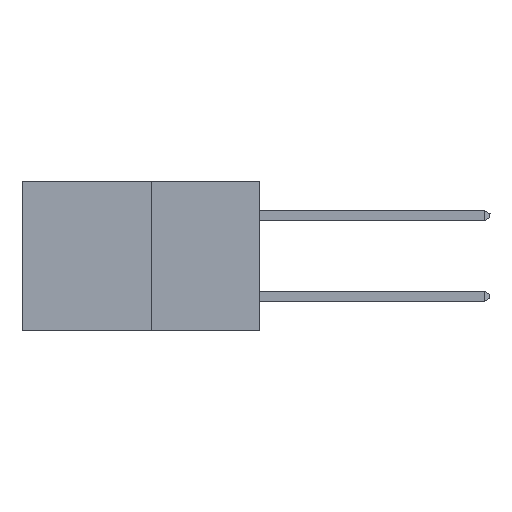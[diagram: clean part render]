
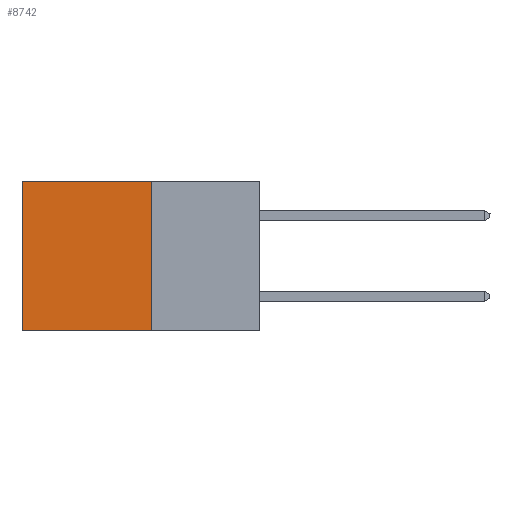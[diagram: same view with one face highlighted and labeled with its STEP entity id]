
A CAD part, left-side view. The second image highlights one B-rep face of the part: STEP entity #8742.
In plain terms, the highlighted planar face has unit normal (-1, 0, 0).
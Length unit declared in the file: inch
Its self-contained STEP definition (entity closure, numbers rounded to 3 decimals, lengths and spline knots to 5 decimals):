
#22 = VECTOR ( 'NONE', #3470, 39.37008 ) ;
#344 = ORIENTED_EDGE ( 'NONE', *, *, #5314, .F. ) ;
#728 = CARTESIAN_POINT ( 'NONE',  ( 0.277, 0.27, -0.37 ) ) ;
#1146 = CARTESIAN_POINT ( 'NONE',  ( 0.277, 0.27, 0. ) ) ;
#1291 = CARTESIAN_POINT ( 'NONE',  ( 0.277, 0.59, 0. ) ) ;
#1607 = VERTEX_POINT ( 'NONE', #6024 ) ;
#1720 = AXIS2_PLACEMENT_3D ( 'NONE', #8151, #7889, #7860 ) ;
#1798 = LINE ( 'NONE', #9121, #11378 ) ;
#2206 = EDGE_CURVE ( 'NONE', #5374, #1607, #2498, .T. ) ;
#2498 = LINE ( 'NONE', #7254, #22 ) ;
#2907 = VERTEX_POINT ( 'NONE', #1146 ) ;
#3053 = DIRECTION ( 'NONE',  ( 0., 0., -1. ) ) ;
#3089 = CARTESIAN_POINT ( 'NONE',  ( 0.277, 0.27, -0.37 ) ) ;
#3358 = ORIENTED_EDGE ( 'NONE', *, *, #2206, .T. ) ;
#3470 = DIRECTION ( 'NONE',  ( 0., 0., -1. ) ) ;
#4469 = LINE ( 'NONE', #3089, #4746 ) ;
#4746 = VECTOR ( 'NONE', #3053, 39.37008 ) ;
#5202 = VERTEX_POINT ( 'NONE', #8430 ) ;
#5314 = EDGE_CURVE ( 'NONE', #5202, #1607, #11297, .T. ) ;
#5374 = VERTEX_POINT ( 'NONE', #1291 ) ;
#6024 = CARTESIAN_POINT ( 'NONE',  ( 0.277, 0.59, -0.37 ) ) ;
#6048 = VECTOR ( 'NONE', #6355, 39.37008 ) ;
#6355 = DIRECTION ( 'NONE',  ( 0., 1., 0. ) ) ;
#6371 = FACE_OUTER_BOUND ( 'NONE', #8436, .T. ) ;
#6474 = EDGE_CURVE ( 'NONE', #2907, #5374, #1798, .T. ) ;
#7254 = CARTESIAN_POINT ( 'NONE',  ( 0.277, 0.59, -0.37 ) ) ;
#7855 = ORIENTED_EDGE ( 'NONE', *, *, #6474, .T. ) ;
#7860 = DIRECTION ( 'NONE',  ( 0., 0., -1. ) ) ;
#7889 = DIRECTION ( 'NONE',  ( 1., 0., 0. ) ) ;
#7947 = PLANE ( 'NONE',  #1720 ) ;
#8151 = CARTESIAN_POINT ( 'NONE',  ( 0.277, 0.27, -0.37 ) ) ;
#8430 = CARTESIAN_POINT ( 'NONE',  ( 0.277, 0.27, -0.37 ) ) ;
#8436 = EDGE_LOOP ( 'NONE', ( #3358, #344, #10543, #7855 ) ) ;
#8742 = ADVANCED_FACE ( 'NONE', ( #6371 ), #7947, .F. ) ;
#9121 = CARTESIAN_POINT ( 'NONE',  ( 0.277, 0.27, 0. ) ) ;
#9154 = EDGE_CURVE ( 'NONE', #2907, #5202, #4469, .T. ) ;
#10543 = ORIENTED_EDGE ( 'NONE', *, *, #9154, .F. ) ;
#10618 = DIRECTION ( 'NONE',  ( 0., 1., 0. ) ) ;
#11297 = LINE ( 'NONE', #728, #6048 ) ;
#11378 = VECTOR ( 'NONE', #10618, 39.37008 ) ;
